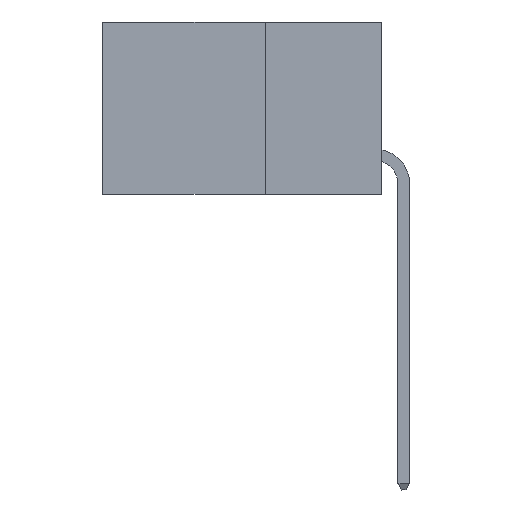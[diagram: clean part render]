
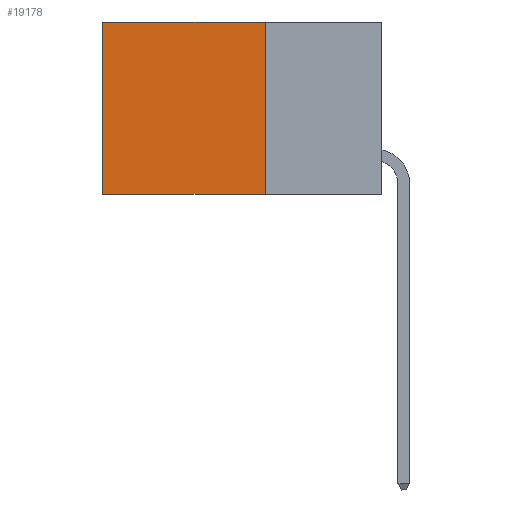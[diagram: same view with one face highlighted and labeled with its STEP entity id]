
A CAD part, left-side view. The second image highlights one B-rep face of the part: STEP entity #19178.
In plain terms, the highlighted planar face has unit normal (-1, 0, 0).
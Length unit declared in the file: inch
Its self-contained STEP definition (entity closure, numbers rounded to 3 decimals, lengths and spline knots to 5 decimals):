
#553 = LINE ( 'NONE', #9135, #15010 ) ;
#793 = LINE ( 'NONE', #14412, #4606 ) ;
#1900 = CARTESIAN_POINT ( 'NONE',  ( 0.2875, 0.6, 0. ) ) ;
#2046 = LINE ( 'NONE', #1900, #20773 ) ;
#2243 = EDGE_CURVE ( 'NONE', #18945, #10021, #793, .T. ) ;
#2478 = VERTEX_POINT ( 'NONE', #4531 ) ;
#3736 = DIRECTION ( 'NONE',  ( 0., 0., -1. ) ) ;
#4531 = CARTESIAN_POINT ( 'NONE',  ( 0.2875, 0.6, -0.37 ) ) ;
#4606 = VECTOR ( 'NONE', #20979, 39.37008 ) ;
#5011 = DIRECTION ( 'NONE',  ( 0., 1., 0. ) ) ;
#5098 = CARTESIAN_POINT ( 'NONE',  ( 0.2875, 0.25, -0.37 ) ) ;
#5186 = ORIENTED_EDGE ( 'NONE', *, *, #2243, .T. ) ;
#5246 = ORIENTED_EDGE ( 'NONE', *, *, #11535, .F. ) ;
#5435 = EDGE_LOOP ( 'NONE', ( #22535, #9291, #5246, #5186 ) ) ;
#6354 = DIRECTION ( 'NONE',  ( 1., 0., 0. ) ) ;
#7545 = CARTESIAN_POINT ( 'NONE',  ( 0.2875, 0.25, 0. ) ) ;
#7637 = LINE ( 'NONE', #5098, #21918 ) ;
#9135 = CARTESIAN_POINT ( 'NONE',  ( 0.2875, 0.25, 0. ) ) ;
#9236 = FACE_OUTER_BOUND ( 'NONE', #5435, .T. ) ;
#9291 = ORIENTED_EDGE ( 'NONE', *, *, #21187, .F. ) ;
#10021 = VERTEX_POINT ( 'NONE', #11811 ) ;
#10684 = VERTEX_POINT ( 'NONE', #15934 ) ;
#11015 = DIRECTION ( 'NONE',  ( 0., 0., -1. ) ) ;
#11535 = EDGE_CURVE ( 'NONE', #18945, #10684, #553, .T. ) ;
#11738 = AXIS2_PLACEMENT_3D ( 'NONE', #17597, #6354, #19437 ) ;
#11811 = CARTESIAN_POINT ( 'NONE',  ( 0.2875, 0.6, 0. ) ) ;
#11903 = PLANE ( 'NONE',  #11738 ) ;
#14412 = CARTESIAN_POINT ( 'NONE',  ( 0.2875, 0.25, 0. ) ) ;
#15010 = VECTOR ( 'NONE', #11015, 39.37008 ) ;
#15934 = CARTESIAN_POINT ( 'NONE',  ( 0.2875, 0.25, -0.37 ) ) ;
#16528 = EDGE_CURVE ( 'NONE', #10021, #2478, #2046, .T. ) ;
#17597 = CARTESIAN_POINT ( 'NONE',  ( 0.2875, 0.25, 0. ) ) ;
#18945 = VERTEX_POINT ( 'NONE', #7545 ) ;
#19178 = ADVANCED_FACE ( 'NONE', ( #9236 ), #11903, .F. ) ;
#19437 = DIRECTION ( 'NONE',  ( 0., 0., -1. ) ) ;
#20773 = VECTOR ( 'NONE', #3736, 39.37008 ) ;
#20979 = DIRECTION ( 'NONE',  ( 0., 1., 0. ) ) ;
#21187 = EDGE_CURVE ( 'NONE', #10684, #2478, #7637, .T. ) ;
#21918 = VECTOR ( 'NONE', #5011, 39.37008 ) ;
#22535 = ORIENTED_EDGE ( 'NONE', *, *, #16528, .T. ) ;
